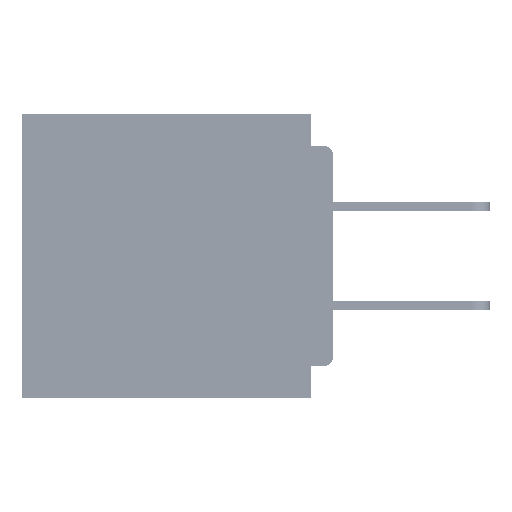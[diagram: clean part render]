
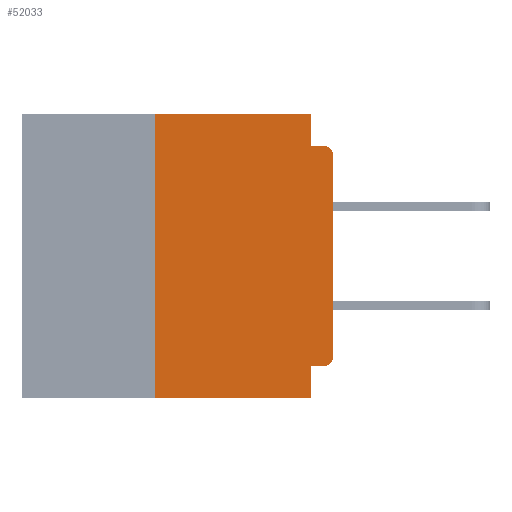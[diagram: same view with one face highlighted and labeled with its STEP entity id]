
A CAD part, left-side view. The second image highlights one B-rep face of the part: STEP entity #52033.
In plain terms, the highlighted planar face has unit normal (-1, 0, 0).
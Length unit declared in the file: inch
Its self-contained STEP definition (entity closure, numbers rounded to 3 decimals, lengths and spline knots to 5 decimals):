
#77 = VERTEX_POINT ( 'NONE', #17718 ) ;
#1410 = VECTOR ( 'NONE', #36723, 39.37008 ) ;
#2286 = ORIENTED_EDGE ( 'NONE', *, *, #40689, .F. ) ;
#2563 = VERTEX_POINT ( 'NONE', #16346 ) ;
#2965 = ORIENTED_EDGE ( 'NONE', *, *, #55617, .T. ) ;
#3138 = DIRECTION ( 'NONE',  ( 0., 0., 1. ) ) ;
#3677 = CARTESIAN_POINT ( 'NONE',  ( 0., 0.031, -0.4 ) ) ;
#4196 = LINE ( 'NONE', #52540, #58459 ) ;
#4285 = DIRECTION ( 'NONE',  ( 0., 0., -1. ) ) ;
#6096 = VERTEX_POINT ( 'NONE', #69404 ) ;
#7724 = LINE ( 'NONE', #55891, #36607 ) ;
#7774 = CARTESIAN_POINT ( 'NONE',  ( 0., 0.25, -0.4 ) ) ;
#8071 = ORIENTED_EDGE ( 'NONE', *, *, #56564, .F. ) ;
#10721 = AXIS2_PLACEMENT_3D ( 'NONE', #69142, #36792, #4285 ) ;
#13478 = CARTESIAN_POINT ( 'NONE',  ( 0., 0.031, -0.4 ) ) ;
#14592 = VERTEX_POINT ( 'NONE', #38212 ) ;
#15610 = ORIENTED_EDGE ( 'NONE', *, *, #25258, .T. ) ;
#15823 = EDGE_CURVE ( 'NONE', #2563, #6096, #61770, .T. ) ;
#16346 = CARTESIAN_POINT ( 'NONE',  ( 0., 0.031, -0.045 ) ) ;
#16800 = CARTESIAN_POINT ( 'NONE',  ( 0., 0.031, -0.355 ) ) ;
#17220 = DIRECTION ( 'NONE',  ( 0., -1., 0. ) ) ;
#17718 = CARTESIAN_POINT ( 'NONE',  ( 0., 0.25, -0.4 ) ) ;
#19394 = CIRCLE ( 'NONE', #37261, 0.015 ) ;
#21451 = EDGE_CURVE ( 'NONE', #54546, #2563, #59124, .T. ) ;
#22645 = CARTESIAN_POINT ( 'NONE',  ( 0., 0., -0.355 ) ) ;
#22666 = CARTESIAN_POINT ( 'NONE',  ( 0., 0., -0.045 ) ) ;
#24539 = LINE ( 'NONE', #22645, #38927 ) ;
#24711 = VECTOR ( 'NONE', #29891, 39.37008 ) ;
#25258 = EDGE_CURVE ( 'NONE', #64458, #46670, #26488, .T. ) ;
#25738 = CARTESIAN_POINT ( 'NONE',  ( 0., 0.015, -0.06 ) ) ;
#25986 = ORIENTED_EDGE ( 'NONE', *, *, #63970, .F. ) ;
#26020 = CARTESIAN_POINT ( 'NONE',  ( 0., 0.437, 0. ) ) ;
#26488 = LINE ( 'NONE', #41088, #55248 ) ;
#26586 = VERTEX_POINT ( 'NONE', #3677 ) ;
#26998 = LINE ( 'NONE', #7774, #66731 ) ;
#27065 = CARTESIAN_POINT ( 'NONE',  ( 0., 0.031, 0. ) ) ;
#27224 = VERTEX_POINT ( 'NONE', #37315 ) ;
#28117 = DIRECTION ( 'NONE',  ( 0., 1., 0. ) ) ;
#29891 = DIRECTION ( 'NONE',  ( 0., 0., -1. ) ) ;
#31188 = DIRECTION ( 'NONE',  ( 0., 0., -1. ) ) ;
#31482 = DIRECTION ( 'NONE',  ( 0., 0., -1. ) ) ;
#35263 = AXIS2_PLACEMENT_3D ( 'NONE', #26020, #63860, #31482 ) ;
#36607 = VECTOR ( 'NONE', #61359, 39.37008 ) ;
#36723 = DIRECTION ( 'NONE',  ( 0., 0., -1. ) ) ;
#36792 = DIRECTION ( 'NONE',  ( -1., 0., 0. ) ) ;
#37261 = AXIS2_PLACEMENT_3D ( 'NONE', #25738, #63580, #31188 ) ;
#37315 = CARTESIAN_POINT ( 'NONE',  ( 0., 0.015, -0.355 ) ) ;
#38049 = ORIENTED_EDGE ( 'NONE', *, *, #54983, .T. ) ;
#38212 = CARTESIAN_POINT ( 'NONE',  ( 0., 0.25, 0. ) ) ;
#38927 = VECTOR ( 'NONE', #28117, 39.37008 ) ;
#39093 = LINE ( 'NONE', #13478, #24711 ) ;
#39868 = EDGE_LOOP ( 'NONE', ( #15610, #2965, #42256, #56832, #59770, #8071, #38049, #2286, #25986, #60480 ) ) ;
#40575 = EDGE_CURVE ( 'NONE', #14592, #54546, #7724, .T. ) ;
#40689 = EDGE_CURVE ( 'NONE', #69950, #26586, #39093, .T. ) ;
#41088 = CARTESIAN_POINT ( 'NONE',  ( 0., 0., 0. ) ) ;
#42256 = ORIENTED_EDGE ( 'NONE', *, *, #15823, .F. ) ;
#43032 = CIRCLE ( 'NONE', #10721, 0.015 ) ;
#45684 = VECTOR ( 'NONE', #17220, 39.37008 ) ;
#46670 = VERTEX_POINT ( 'NONE', #63172 ) ;
#52033 = ADVANCED_FACE ( 'NONE', ( #68155 ), #52998, .F. ) ;
#52540 = CARTESIAN_POINT ( 'NONE',  ( 0., 0.437, -0.4 ) ) ;
#52998 = PLANE ( 'NONE',  #35263 ) ;
#54546 = VERTEX_POINT ( 'NONE', #27065 ) ;
#54983 = EDGE_CURVE ( 'NONE', #77, #26586, #4196, .T. ) ;
#55248 = VECTOR ( 'NONE', #3138, 39.37008 ) ;
#55617 = EDGE_CURVE ( 'NONE', #46670, #6096, #19394, .T. ) ;
#55891 = CARTESIAN_POINT ( 'NONE',  ( 0., 0.437, 0. ) ) ;
#56344 = DIRECTION ( 'NONE',  ( 0., 0., 1. ) ) ;
#56564 = EDGE_CURVE ( 'NONE', #77, #14592, #26998, .T. ) ;
#56832 = ORIENTED_EDGE ( 'NONE', *, *, #21451, .F. ) ;
#58002 = DIRECTION ( 'NONE',  ( 0., -1., 0. ) ) ;
#58459 = VECTOR ( 'NONE', #58002, 39.37008 ) ;
#59124 = LINE ( 'NONE', #63668, #1410 ) ;
#59770 = ORIENTED_EDGE ( 'NONE', *, *, #40575, .F. ) ;
#60480 = ORIENTED_EDGE ( 'NONE', *, *, #69202, .T. ) ;
#61359 = DIRECTION ( 'NONE',  ( 0., -1., 0. ) ) ;
#61770 = LINE ( 'NONE', #22666, #45684 ) ;
#63172 = CARTESIAN_POINT ( 'NONE',  ( 0., 0., -0.06 ) ) ;
#63580 = DIRECTION ( 'NONE',  ( -1., 0., 0. ) ) ;
#63668 = CARTESIAN_POINT ( 'NONE',  ( 0., 0.031, 0. ) ) ;
#63860 = DIRECTION ( 'NONE',  ( 1., 0., 0. ) ) ;
#63970 = EDGE_CURVE ( 'NONE', #27224, #69950, #24539, .T. ) ;
#64458 = VERTEX_POINT ( 'NONE', #70091 ) ;
#66731 = VECTOR ( 'NONE', #56344, 39.37008 ) ;
#68155 = FACE_OUTER_BOUND ( 'NONE', #39868, .T. ) ;
#69142 = CARTESIAN_POINT ( 'NONE',  ( 0., 0.015, -0.34 ) ) ;
#69202 = EDGE_CURVE ( 'NONE', #27224, #64458, #43032, .T. ) ;
#69404 = CARTESIAN_POINT ( 'NONE',  ( 0., 0.015, -0.045 ) ) ;
#69950 = VERTEX_POINT ( 'NONE', #16800 ) ;
#70091 = CARTESIAN_POINT ( 'NONE',  ( 0., 0., -0.34 ) ) ;
